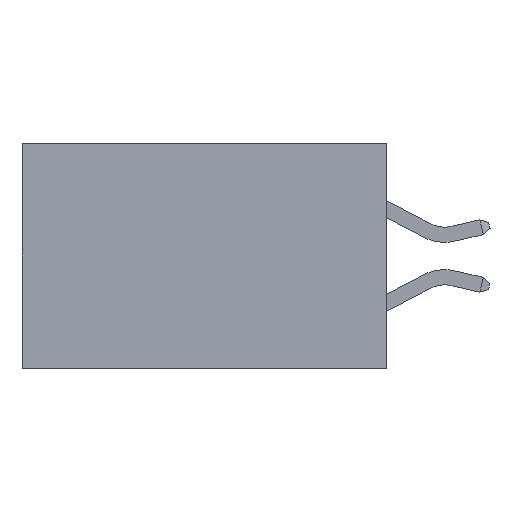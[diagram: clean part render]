
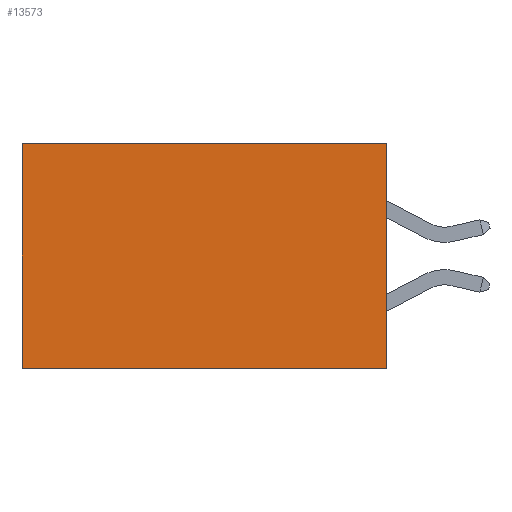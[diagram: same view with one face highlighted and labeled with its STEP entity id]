
A CAD part, left-side view. The second image highlights one B-rep face of the part: STEP entity #13573.
In plain terms, the highlighted planar face has unit normal (-1, 0, 0).
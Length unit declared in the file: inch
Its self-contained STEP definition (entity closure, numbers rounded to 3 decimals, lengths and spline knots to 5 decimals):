
#945 = VERTEX_POINT ( 'NONE', #4076 ) ;
#1431 = CARTESIAN_POINT ( 'NONE',  ( 0.298, 0., -0.37 ) ) ;
#1619 = EDGE_CURVE ( 'NONE', #945, #9008, #3668, .T. ) ;
#2529 = DIRECTION ( 'NONE',  ( 0., 1., 0. ) ) ;
#2540 = EDGE_LOOP ( 'NONE', ( #15984, #4597, #18073, #12604 ) ) ;
#3122 = VECTOR ( 'NONE', #2529, 39.37008 ) ;
#3349 = LINE ( 'NONE', #17271, #17112 ) ;
#3607 = VERTEX_POINT ( 'NONE', #4268 ) ;
#3668 = LINE ( 'NONE', #14936, #3122 ) ;
#4076 = CARTESIAN_POINT ( 'NONE',  ( 0.298, 0., 0. ) ) ;
#4268 = CARTESIAN_POINT ( 'NONE',  ( 0.298, 0., -0.37 ) ) ;
#4597 = ORIENTED_EDGE ( 'NONE', *, *, #13169, .F. ) ;
#5460 = AXIS2_PLACEMENT_3D ( 'NONE', #16228, #5908, #17907 ) ;
#5908 = DIRECTION ( 'NONE',  ( 1., 0., 0. ) ) ;
#8637 = CARTESIAN_POINT ( 'NONE',  ( 0.298, 0., 0. ) ) ;
#8817 = CARTESIAN_POINT ( 'NONE',  ( 0.298, 0.6, 0. ) ) ;
#9008 = VERTEX_POINT ( 'NONE', #8817 ) ;
#10300 = VERTEX_POINT ( 'NONE', #14029 ) ;
#10878 = VECTOR ( 'NONE', #22191, 39.37008 ) ;
#11083 = PLANE ( 'NONE',  #5460 ) ;
#11331 = VECTOR ( 'NONE', #16969, 39.37008 ) ;
#12374 = FACE_OUTER_BOUND ( 'NONE', #2540, .T. ) ;
#12604 = ORIENTED_EDGE ( 'NONE', *, *, #1619, .T. ) ;
#13169 = EDGE_CURVE ( 'NONE', #3607, #10300, #15908, .T. ) ;
#13573 = ADVANCED_FACE ( 'NONE', ( #12374 ), #11083, .F. ) ;
#14029 = CARTESIAN_POINT ( 'NONE',  ( 0.298, 0.6, -0.37 ) ) ;
#14936 = CARTESIAN_POINT ( 'NONE',  ( 0.298, 0., 0. ) ) ;
#15908 = LINE ( 'NONE', #1431, #11331 ) ;
#15984 = ORIENTED_EDGE ( 'NONE', *, *, #16130, .T. ) ;
#16130 = EDGE_CURVE ( 'NONE', #9008, #10300, #3349, .T. ) ;
#16228 = CARTESIAN_POINT ( 'NONE',  ( 0.298, 0., 0. ) ) ;
#16969 = DIRECTION ( 'NONE',  ( 0., 1., 0. ) ) ;
#17112 = VECTOR ( 'NONE', #17334, 39.37008 ) ;
#17271 = CARTESIAN_POINT ( 'NONE',  ( 0.298, 0.6, 0. ) ) ;
#17334 = DIRECTION ( 'NONE',  ( 0., 0., -1. ) ) ;
#17907 = DIRECTION ( 'NONE',  ( 0., 0., -1. ) ) ;
#18073 = ORIENTED_EDGE ( 'NONE', *, *, #18839, .F. ) ;
#18839 = EDGE_CURVE ( 'NONE', #945, #3607, #20390, .T. ) ;
#20390 = LINE ( 'NONE', #8637, #10878 ) ;
#22191 = DIRECTION ( 'NONE',  ( 0., 0., -1. ) ) ;
